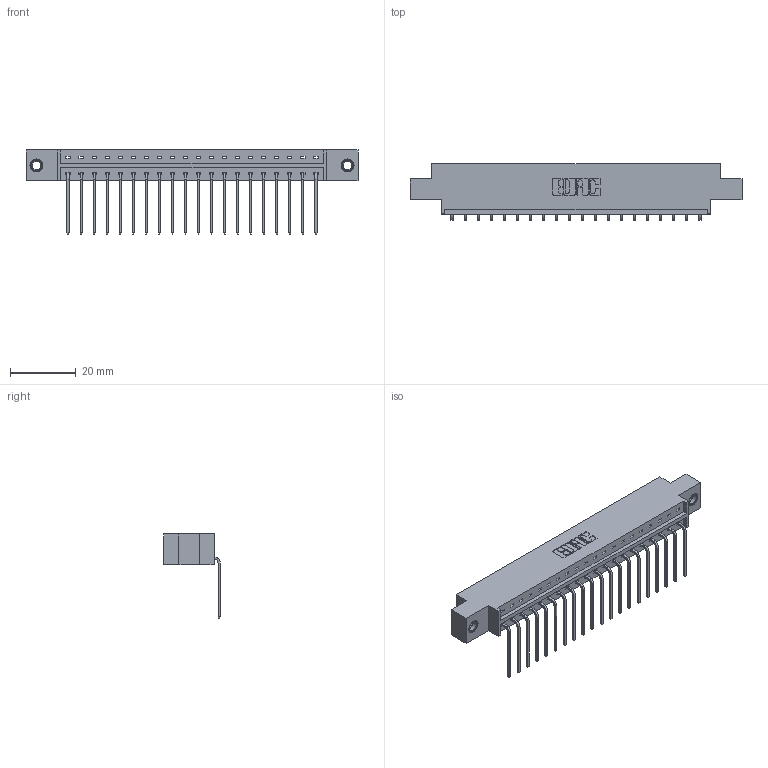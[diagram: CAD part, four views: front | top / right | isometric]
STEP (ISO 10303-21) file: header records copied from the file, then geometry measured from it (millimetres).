
FILE_DESCRIPTION (( 'STEP AP203' ), '1' );
FILE_NAME ('333-020-559-607.STEP', '2018-08-02T00:42:57', ( '' ), ( '' ), 'SwSTEP 2.0', 'SolidWorks 2016', '' );
FILE_SCHEMA (( 'CONFIG_CONTROL_DESIGN' ));
Length unit declared in the file: inch
Products named in the file (4): 333 Part_Offset - .156 Dia - TI; 345-292-001_558 559 Tail - 1; 345-250-001_345-250-005-103; 333-020-559-607
Assembly tree (23 placements, depth 2):
  333-020-559-607
    333 Part_Offset - .156 Dia - TI
    345-292-001_558 559 Tail - 1  x20
    345-250-001_345-250-005-103  x2
Bounding box: 100.79 x 17.09 x 25.53 mm (x, y, z)
Volume: 9778.2 mm3; surface area: 11079.9 mm2
Topology: 23 solids, 23 shells, 1378 faces, 4099 edges, 2698 vertices
Faces by surface type: plane 986, cylinder 376, cone 12, torus 4
Entity records: 16474 total; most frequent: CARTESIAN_POINT 2829, ORIENTED_EDGE 2778, DIRECTION 2463, EDGE_CURVE 1389, VECTOR 1241, LINE 1241, VERTEX_POINT 920, AXIS2_PLACEMENT_3D 611
